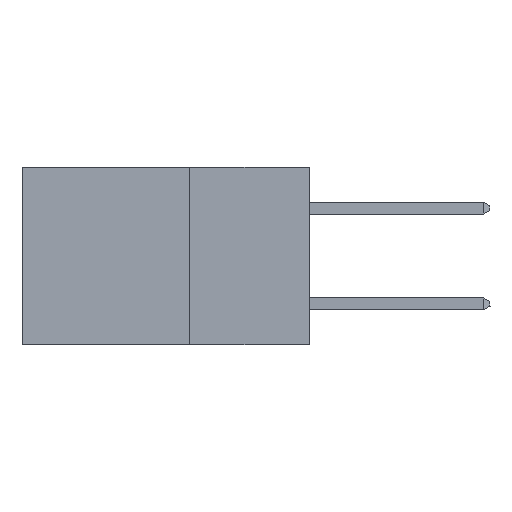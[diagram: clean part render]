
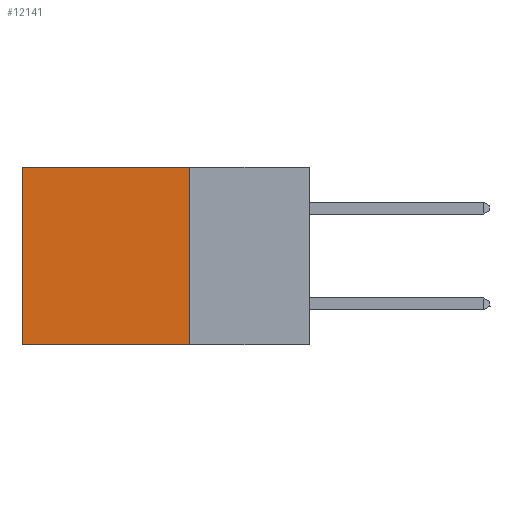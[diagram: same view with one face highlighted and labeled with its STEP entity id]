
A CAD part, left-side view. The second image highlights one B-rep face of the part: STEP entity #12141.
In plain terms, the highlighted planar face has unit normal (-1, 0, 0).
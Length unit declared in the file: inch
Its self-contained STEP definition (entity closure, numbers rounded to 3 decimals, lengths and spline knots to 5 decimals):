
#1075 = DIRECTION ( 'NONE',  ( 1., 0., 0. ) ) ;
#1103 = CARTESIAN_POINT ( 'NONE',  ( 0.2875, 0.25, -0.37 ) ) ;
#1432 = CARTESIAN_POINT ( 'NONE',  ( 0.2875, 0.25, 0. ) ) ;
#2579 = AXIS2_PLACEMENT_3D ( 'NONE', #11936, #1075, #3351 ) ;
#3249 = CARTESIAN_POINT ( 'NONE',  ( 0.2875, 0.25, -0.37 ) ) ;
#3351 = DIRECTION ( 'NONE',  ( 0., 0., -1. ) ) ;
#3469 = VECTOR ( 'NONE', #27525, 39.37008 ) ;
#4897 = LINE ( 'NONE', #19767, #7029 ) ;
#7029 = VECTOR ( 'NONE', #26493, 39.37008 ) ;
#7526 = LINE ( 'NONE', #16250, #12361 ) ;
#7630 = FACE_OUTER_BOUND ( 'NONE', #17277, .T. ) ;
#10145 = DIRECTION ( 'NONE',  ( 0., 1., 0. ) ) ;
#10248 = ORIENTED_EDGE ( 'NONE', *, *, #18928, .T. ) ;
#10686 = CARTESIAN_POINT ( 'NONE',  ( 0.2875, 0.6, 0. ) ) ;
#11545 = ORIENTED_EDGE ( 'NONE', *, *, #25200, .F. ) ;
#11690 = VERTEX_POINT ( 'NONE', #3249 ) ;
#11936 = CARTESIAN_POINT ( 'NONE',  ( 0.2875, 0.25, 0. ) ) ;
#12141 = ADVANCED_FACE ( 'NONE', ( #7630 ), #18778, .F. ) ;
#12361 = VECTOR ( 'NONE', #20687, 39.37008 ) ;
#14815 = ORIENTED_EDGE ( 'NONE', *, *, #14942, .F. ) ;
#14942 = EDGE_CURVE ( 'NONE', #11690, #22097, #20808, .T. ) ;
#16250 = CARTESIAN_POINT ( 'NONE',  ( 0.2875, 0.25, 0. ) ) ;
#17277 = EDGE_LOOP ( 'NONE', ( #20785, #14815, #11545, #10248 ) ) ;
#18135 = EDGE_CURVE ( 'NONE', #26590, #22097, #4897, .T. ) ;
#18778 = PLANE ( 'NONE',  #2579 ) ;
#18815 = VECTOR ( 'NONE', #10145, 39.37008 ) ;
#18928 = EDGE_CURVE ( 'NONE', #20469, #26590, #25583, .T. ) ;
#19767 = CARTESIAN_POINT ( 'NONE',  ( 0.2875, 0.6, 0. ) ) ;
#20469 = VERTEX_POINT ( 'NONE', #24841 ) ;
#20687 = DIRECTION ( 'NONE',  ( 0., 0., -1. ) ) ;
#20785 = ORIENTED_EDGE ( 'NONE', *, *, #18135, .T. ) ;
#20808 = LINE ( 'NONE', #1103, #3469 ) ;
#22097 = VERTEX_POINT ( 'NONE', #25270 ) ;
#24841 = CARTESIAN_POINT ( 'NONE',  ( 0.2875, 0.25, 0. ) ) ;
#25200 = EDGE_CURVE ( 'NONE', #20469, #11690, #7526, .T. ) ;
#25270 = CARTESIAN_POINT ( 'NONE',  ( 0.2875, 0.6, -0.37 ) ) ;
#25583 = LINE ( 'NONE', #1432, #18815 ) ;
#26493 = DIRECTION ( 'NONE',  ( 0., 0., -1. ) ) ;
#26590 = VERTEX_POINT ( 'NONE', #10686 ) ;
#27525 = DIRECTION ( 'NONE',  ( 0., 1., 0. ) ) ;
